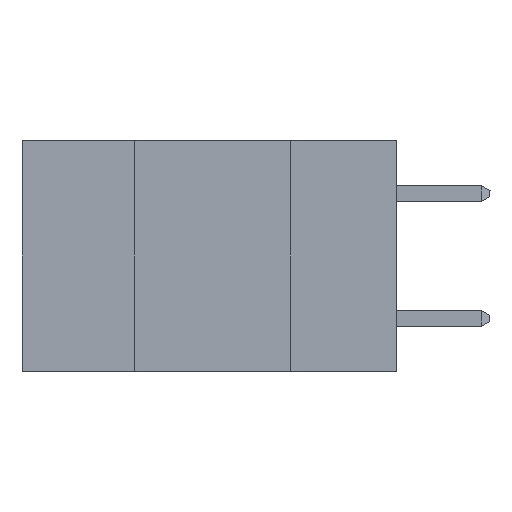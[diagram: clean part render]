
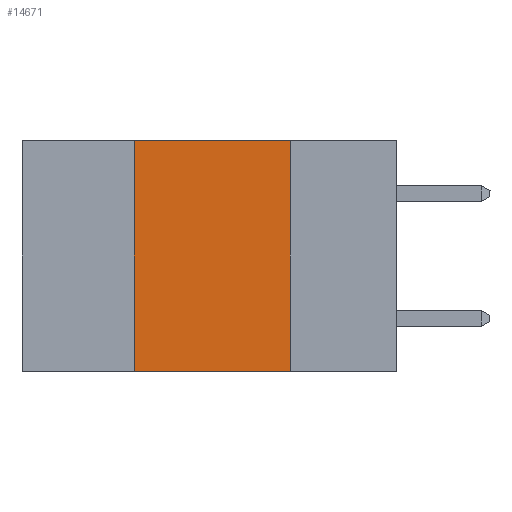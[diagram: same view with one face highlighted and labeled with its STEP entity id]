
A CAD part, left-side view. The second image highlights one B-rep face of the part: STEP entity #14671.
In plain terms, the highlighted planar face has unit normal (-1, 0, 0).
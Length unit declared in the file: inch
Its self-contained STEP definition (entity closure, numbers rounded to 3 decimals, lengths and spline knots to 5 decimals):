
#1407 = VECTOR ( 'NONE', #7703, 39.37008 ) ;
#1460 = DIRECTION ( 'NONE',  ( 1., 0., 0. ) ) ;
#1761 = ORIENTED_EDGE ( 'NONE', *, *, #10695, .F. ) ;
#2540 = VECTOR ( 'NONE', #2683, 39.37008 ) ;
#2683 = DIRECTION ( 'NONE',  ( 0., -1., 0. ) ) ;
#3095 = EDGE_CURVE ( 'NONE', #3318, #3178, #16290, .T. ) ;
#3178 = VERTEX_POINT ( 'NONE', #14642 ) ;
#3318 = VERTEX_POINT ( 'NONE', #9708 ) ;
#4152 = CARTESIAN_POINT ( 'NONE',  ( 0., 0.17, 0. ) ) ;
#4201 = VECTOR ( 'NONE', #11079, 39.37008 ) ;
#4859 = LINE ( 'NONE', #12712, #1407 ) ;
#5449 = EDGE_CURVE ( 'NONE', #7614, #3318, #12683, .T. ) ;
#6007 = CARTESIAN_POINT ( 'NONE',  ( 0., 0.42, 0. ) ) ;
#6584 = CARTESIAN_POINT ( 'NONE',  ( 0., 0.6, 0. ) ) ;
#7062 = EDGE_LOOP ( 'NONE', ( #14300, #8218, #1761, #9084 ) ) ;
#7311 = FACE_OUTER_BOUND ( 'NONE', #7062, .T. ) ;
#7582 = LINE ( 'NONE', #6007, #4201 ) ;
#7614 = VERTEX_POINT ( 'NONE', #9649 ) ;
#7703 = DIRECTION ( 'NONE',  ( 0., -1., 0. ) ) ;
#8218 = ORIENTED_EDGE ( 'NONE', *, *, #5449, .F. ) ;
#9084 = ORIENTED_EDGE ( 'NONE', *, *, #9246, .T. ) ;
#9246 = EDGE_CURVE ( 'NONE', #13960, #3178, #4859, .T. ) ;
#9457 = AXIS2_PLACEMENT_3D ( 'NONE', #11617, #1460, #10413 ) ;
#9649 = CARTESIAN_POINT ( 'NONE',  ( 0., 0.42, 0. ) ) ;
#9708 = CARTESIAN_POINT ( 'NONE',  ( 0., 0.17, 0. ) ) ;
#10413 = DIRECTION ( 'NONE',  ( 0., 0., -1. ) ) ;
#10542 = CARTESIAN_POINT ( 'NONE',  ( 0., 0.42, -0.37 ) ) ;
#10695 = EDGE_CURVE ( 'NONE', #13960, #7614, #7582, .T. ) ;
#11079 = DIRECTION ( 'NONE',  ( 0., 0., 1. ) ) ;
#11617 = CARTESIAN_POINT ( 'NONE',  ( 0., 0.6, 0. ) ) ;
#12683 = LINE ( 'NONE', #6584, #2540 ) ;
#12712 = CARTESIAN_POINT ( 'NONE',  ( 0., 0.6, -0.37 ) ) ;
#13960 = VERTEX_POINT ( 'NONE', #10542 ) ;
#14300 = ORIENTED_EDGE ( 'NONE', *, *, #3095, .F. ) ;
#14642 = CARTESIAN_POINT ( 'NONE',  ( 0., 0.17, -0.37 ) ) ;
#14671 = ADVANCED_FACE ( 'NONE', ( #7311 ), #15400, .F. ) ;
#15400 = PLANE ( 'NONE',  #9457 ) ;
#15893 = VECTOR ( 'NONE', #16294, 39.37008 ) ;
#16290 = LINE ( 'NONE', #4152, #15893 ) ;
#16294 = DIRECTION ( 'NONE',  ( 0., 0., -1. ) ) ;
